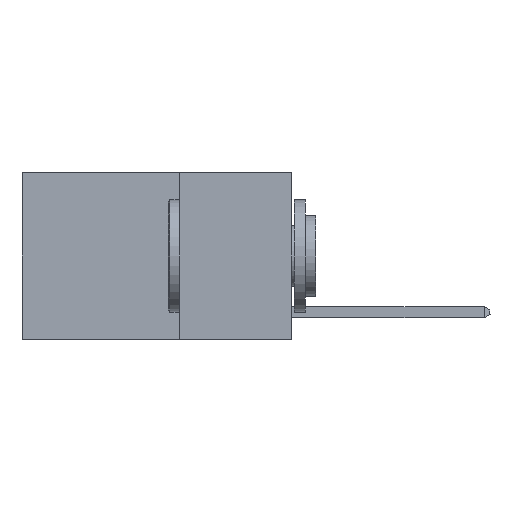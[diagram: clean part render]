
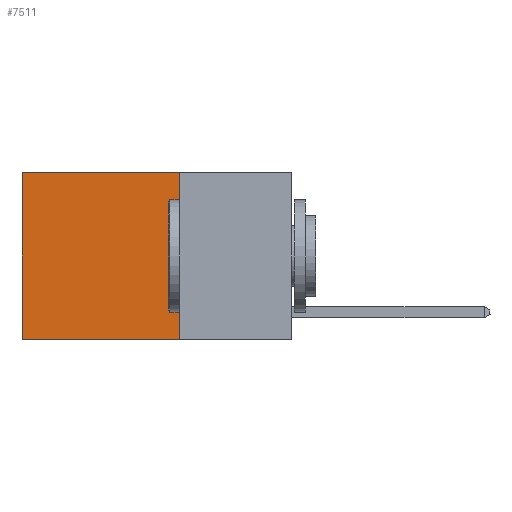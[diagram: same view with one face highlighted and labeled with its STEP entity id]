
A CAD part, left-side view. The second image highlights one B-rep face of the part: STEP entity #7511.
In plain terms, the highlighted planar face has unit normal (-1, 0, 0).
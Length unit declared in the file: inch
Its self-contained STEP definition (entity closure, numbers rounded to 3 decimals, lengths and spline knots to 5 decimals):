
#377 = CARTESIAN_POINT ( 'NONE',  ( 0.2625, 0.6, 0. ) ) ;
#1199 = ORIENTED_EDGE ( 'NONE', *, *, #5243, .T. ) ;
#1463 = LINE ( 'NONE', #2985, #3856 ) ;
#1740 = VERTEX_POINT ( 'NONE', #8760 ) ;
#1890 = VECTOR ( 'NONE', #6139, 39.37008 ) ;
#2382 = EDGE_CURVE ( 'NONE', #4267, #5941, #1463, .T. ) ;
#2594 = LINE ( 'NONE', #3207, #1890 ) ;
#2985 = CARTESIAN_POINT ( 'NONE',  ( 0.2625, 0.6, 0. ) ) ;
#3044 = LINE ( 'NONE', #3892, #3905 ) ;
#3087 = DIRECTION ( 'NONE',  ( 0., 0., -1. ) ) ;
#3093 = DIRECTION ( 'NONE',  ( 1., 0., 0. ) ) ;
#3207 = CARTESIAN_POINT ( 'NONE',  ( 0.2625, 0.25, -0.37 ) ) ;
#3504 = VERTEX_POINT ( 'NONE', #4544 ) ;
#3806 = DIRECTION ( 'NONE',  ( 0., 0., -1. ) ) ;
#3856 = VECTOR ( 'NONE', #8948, 39.37008 ) ;
#3892 = CARTESIAN_POINT ( 'NONE',  ( 0.2625, 0.25, 0. ) ) ;
#3905 = VECTOR ( 'NONE', #3087, 39.37008 ) ;
#4267 = VERTEX_POINT ( 'NONE', #377 ) ;
#4409 = LINE ( 'NONE', #9656, #9349 ) ;
#4484 = EDGE_CURVE ( 'NONE', #1740, #3504, #3044, .T. ) ;
#4544 = CARTESIAN_POINT ( 'NONE',  ( 0.2625, 0.25, -0.37 ) ) ;
#5053 = EDGE_CURVE ( 'NONE', #3504, #5941, #2594, .T. ) ;
#5243 = EDGE_CURVE ( 'NONE', #1740, #4267, #4409, .T. ) ;
#5563 = CARTESIAN_POINT ( 'NONE',  ( 0.2625, 0.6, -0.37 ) ) ;
#5764 = EDGE_LOOP ( 'NONE', ( #7688, #8857, #8303, #1199 ) ) ;
#5941 = VERTEX_POINT ( 'NONE', #5563 ) ;
#5971 = PLANE ( 'NONE',  #9197 ) ;
#6139 = DIRECTION ( 'NONE',  ( 0., 1., 0. ) ) ;
#7328 = FACE_OUTER_BOUND ( 'NONE', #5764, .T. ) ;
#7511 = ADVANCED_FACE ( 'NONE', ( #7328 ), #5971, .F. ) ;
#7688 = ORIENTED_EDGE ( 'NONE', *, *, #2382, .T. ) ;
#8303 = ORIENTED_EDGE ( 'NONE', *, *, #4484, .F. ) ;
#8760 = CARTESIAN_POINT ( 'NONE',  ( 0.2625, 0.25, 0. ) ) ;
#8857 = ORIENTED_EDGE ( 'NONE', *, *, #5053, .F. ) ;
#8878 = DIRECTION ( 'NONE',  ( 0., 1., 0. ) ) ;
#8948 = DIRECTION ( 'NONE',  ( 0., 0., -1. ) ) ;
#8961 = CARTESIAN_POINT ( 'NONE',  ( 0.2625, 0.25, 0. ) ) ;
#9197 = AXIS2_PLACEMENT_3D ( 'NONE', #8961, #3093, #3806 ) ;
#9349 = VECTOR ( 'NONE', #8878, 39.37008 ) ;
#9656 = CARTESIAN_POINT ( 'NONE',  ( 0.2625, 0.25, 0. ) ) ;
